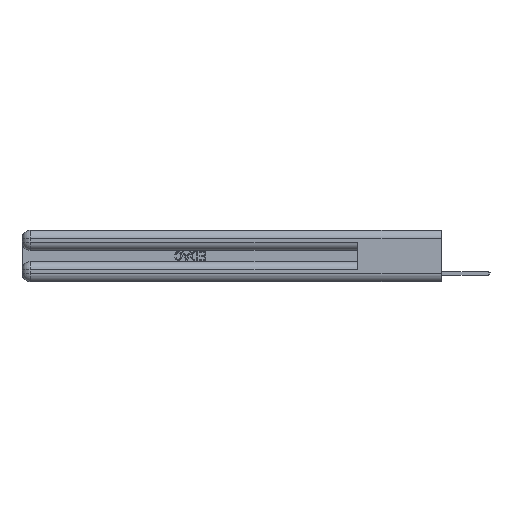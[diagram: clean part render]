
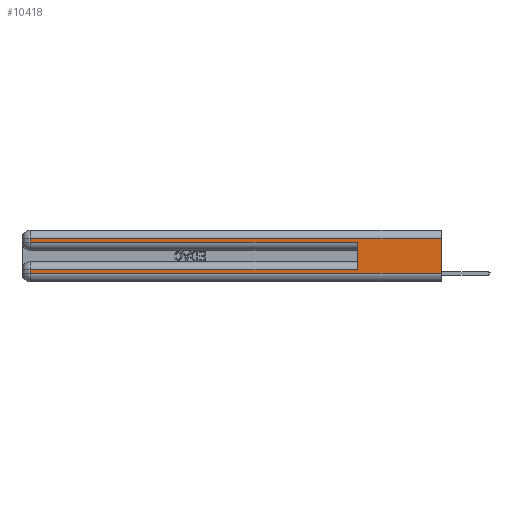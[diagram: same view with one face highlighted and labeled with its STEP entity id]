
A CAD part, left-side view. The second image highlights one B-rep face of the part: STEP entity #10418.
In plain terms, the highlighted planar face has unit normal (-1, 0, 0).
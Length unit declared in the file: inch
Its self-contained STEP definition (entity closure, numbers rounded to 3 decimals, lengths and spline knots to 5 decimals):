
#111 = VERTEX_POINT ( 'NONE', #8996 ) ;
#206 = CARTESIAN_POINT ( 'NONE',  ( 0., 2.94, 0.31 ) ) ;
#915 = VECTOR ( 'NONE', #23769, 39.37008 ) ;
#1383 = VERTEX_POINT ( 'NONE', #21308 ) ;
#1418 = DIRECTION ( 'NONE',  ( 0., 0., -1. ) ) ;
#1575 = CARTESIAN_POINT ( 'NONE',  ( 0., 2.94, 0.285 ) ) ;
#1906 = CARTESIAN_POINT ( 'NONE',  ( 0., 2.94, 0.06 ) ) ;
#2181 = FACE_OUTER_BOUND ( 'NONE', #26198, .T. ) ;
#2201 = VECTOR ( 'NONE', #19622, 39.37008 ) ;
#2579 = CARTESIAN_POINT ( 'NONE',  ( 0., 0., 0.285 ) ) ;
#2624 = EDGE_CURVE ( 'NONE', #23267, #111, #20037, .T. ) ;
#2627 = CARTESIAN_POINT ( 'NONE',  ( 0., 2.94, 0.37 ) ) ;
#3182 = EDGE_CURVE ( 'NONE', #3735, #23267, #5213, .T. ) ;
#3629 = LINE ( 'NONE', #18687, #7828 ) ;
#3672 = VERTEX_POINT ( 'NONE', #11901 ) ;
#3735 = VERTEX_POINT ( 'NONE', #206 ) ;
#3822 = VERTEX_POINT ( 'NONE', #1906 ) ;
#4007 = ORIENTED_EDGE ( 'NONE', *, *, #3182, .T. ) ;
#5125 = VECTOR ( 'NONE', #21001, 39.37008 ) ;
#5213 = LINE ( 'NONE', #14083, #26810 ) ;
#5507 = ORIENTED_EDGE ( 'NONE', *, *, #18213, .T. ) ;
#5924 = ORIENTED_EDGE ( 'NONE', *, *, #22073, .T. ) ;
#6970 = EDGE_CURVE ( 'NONE', #3672, #111, #10146, .T. ) ;
#6980 = LINE ( 'NONE', #2627, #9175 ) ;
#7138 = LINE ( 'NONE', #15737, #23888 ) ;
#7641 = EDGE_CURVE ( 'NONE', #3822, #1383, #3629, .T. ) ;
#7828 = VECTOR ( 'NONE', #18964, 39.37008 ) ;
#8149 = VERTEX_POINT ( 'NONE', #9973 ) ;
#8634 = CARTESIAN_POINT ( 'NONE',  ( 0., 0., 0.37 ) ) ;
#8996 = CARTESIAN_POINT ( 'NONE',  ( 0., 0.6, 0.285 ) ) ;
#9175 = VECTOR ( 'NONE', #13313, 39.37008 ) ;
#9519 = DIRECTION ( 'NONE',  ( 0., 1., 0. ) ) ;
#9973 = CARTESIAN_POINT ( 'NONE',  ( 0., 0., 0.31 ) ) ;
#10146 = LINE ( 'NONE', #18755, #5125 ) ;
#10418 = ADVANCED_FACE ( 'NONE', ( #2181 ), #10754, .F. ) ;
#10514 = ORIENTED_EDGE ( 'NONE', *, *, #15210, .T. ) ;
#10754 = PLANE ( 'NONE',  #16028 ) ;
#11901 = CARTESIAN_POINT ( 'NONE',  ( 0., 0.6, 0.085 ) ) ;
#12921 = LINE ( 'NONE', #21794, #915 ) ;
#13177 = ORIENTED_EDGE ( 'NONE', *, *, #6970, .F. ) ;
#13313 = DIRECTION ( 'NONE',  ( 0., 0., -1. ) ) ;
#14083 = CARTESIAN_POINT ( 'NONE',  ( 0., 2.94, 0.37 ) ) ;
#14636 = CARTESIAN_POINT ( 'NONE',  ( 0., 2.94, 0.085 ) ) ;
#15198 = LINE ( 'NONE', #23239, #26988 ) ;
#15210 = EDGE_CURVE ( 'NONE', #3672, #20111, #12921, .T. ) ;
#15737 = CARTESIAN_POINT ( 'NONE',  ( 0., 0., 0.31 ) ) ;
#16028 = AXIS2_PLACEMENT_3D ( 'NONE', #8634, #17241, #25823 ) ;
#16768 = DIRECTION ( 'NONE',  ( 0., 0., -1. ) ) ;
#17241 = DIRECTION ( 'NONE',  ( 1., 0., 0. ) ) ;
#18213 = EDGE_CURVE ( 'NONE', #8149, #3735, #7138, .T. ) ;
#18687 = CARTESIAN_POINT ( 'NONE',  ( 0., 0., 0.06 ) ) ;
#18755 = CARTESIAN_POINT ( 'NONE',  ( 0., 0.6, 0.145 ) ) ;
#18964 = DIRECTION ( 'NONE',  ( 0., -1., 0. ) ) ;
#19622 = DIRECTION ( 'NONE',  ( 0., -1., 0. ) ) ;
#20037 = LINE ( 'NONE', #2579, #2201 ) ;
#20111 = VERTEX_POINT ( 'NONE', #14636 ) ;
#20986 = ORIENTED_EDGE ( 'NONE', *, *, #7641, .T. ) ;
#21001 = DIRECTION ( 'NONE',  ( 0., 0., 1. ) ) ;
#21308 = CARTESIAN_POINT ( 'NONE',  ( 0., 0., 0.06 ) ) ;
#21794 = CARTESIAN_POINT ( 'NONE',  ( 0., 0., 0.085 ) ) ;
#22073 = EDGE_CURVE ( 'NONE', #20111, #3822, #6980, .T. ) ;
#23239 = CARTESIAN_POINT ( 'NONE',  ( 0., 0., 0.37 ) ) ;
#23267 = VERTEX_POINT ( 'NONE', #1575 ) ;
#23769 = DIRECTION ( 'NONE',  ( 0., 1., 0. ) ) ;
#23888 = VECTOR ( 'NONE', #9519, 39.37008 ) ;
#24826 = EDGE_CURVE ( 'NONE', #8149, #1383, #15198, .T. ) ;
#25698 = ORIENTED_EDGE ( 'NONE', *, *, #2624, .T. ) ;
#25823 = DIRECTION ( 'NONE',  ( 0., 0., -1. ) ) ;
#26198 = EDGE_LOOP ( 'NONE', ( #26406, #5507, #4007, #25698, #13177, #10514, #5924, #20986 ) ) ;
#26406 = ORIENTED_EDGE ( 'NONE', *, *, #24826, .F. ) ;
#26810 = VECTOR ( 'NONE', #1418, 39.37008 ) ;
#26988 = VECTOR ( 'NONE', #16768, 39.37008 ) ;
